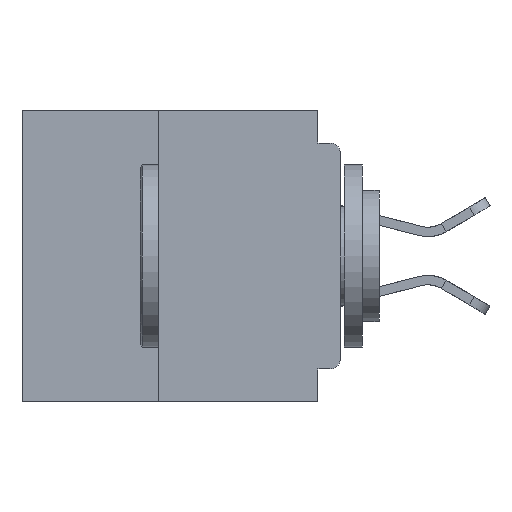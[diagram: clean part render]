
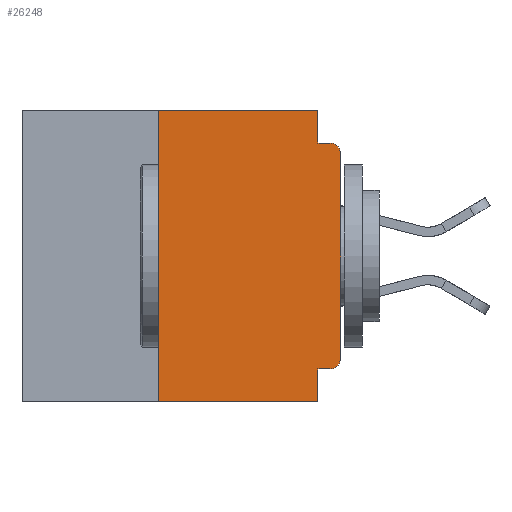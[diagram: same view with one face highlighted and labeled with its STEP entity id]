
A CAD part, left-side view. The second image highlights one B-rep face of the part: STEP entity #26248.
In plain terms, the highlighted planar face has unit normal (-1, 0, 0).
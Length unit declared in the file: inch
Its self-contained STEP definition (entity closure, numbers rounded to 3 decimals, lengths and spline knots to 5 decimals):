
#194 = CARTESIAN_POINT ( 'NONE',  ( 0., 0.031, 0. ) ) ;
#1100 = EDGE_CURVE ( 'NONE', #18490, #32679, #35840, .T. ) ;
#1184 = CARTESIAN_POINT ( 'NONE',  ( 0., 0.031, -0.355 ) ) ;
#1563 = LINE ( 'NONE', #12552, #19149 ) ;
#1639 = EDGE_CURVE ( 'NONE', #33108, #32679, #39386, .T. ) ;
#1641 = DIRECTION ( 'NONE',  ( 0., 0., 1. ) ) ;
#1700 = CIRCLE ( 'NONE', #5880, 0.015 ) ;
#2283 = AXIS2_PLACEMENT_3D ( 'NONE', #19718, #26554, #42294 ) ;
#2343 = EDGE_LOOP ( 'NONE', ( #5915, #18341, #32738, #18912, #7862, #12499, #14066, #38312, #11732, #7358 ) ) ;
#3654 = CARTESIAN_POINT ( 'NONE',  ( 0., 0., -0.06 ) ) ;
#3846 = EDGE_CURVE ( 'NONE', #9332, #11466, #1563, .T. ) ;
#4292 = LINE ( 'NONE', #27196, #38359 ) ;
#5550 = LINE ( 'NONE', #24777, #30886 ) ;
#5880 = AXIS2_PLACEMENT_3D ( 'NONE', #35797, #16117, #39102 ) ;
#5915 = ORIENTED_EDGE ( 'NONE', *, *, #14780, .T. ) ;
#7035 = LINE ( 'NONE', #39237, #15912 ) ;
#7358 = ORIENTED_EDGE ( 'NONE', *, *, #35491, .T. ) ;
#7862 = ORIENTED_EDGE ( 'NONE', *, *, #12087, .F. ) ;
#8947 = VECTOR ( 'NONE', #26849, 39.37008 ) ;
#9332 = VERTEX_POINT ( 'NONE', #1184 ) ;
#9458 = DIRECTION ( 'NONE',  ( 0., 0., 1. ) ) ;
#10410 = PLANE ( 'NONE',  #27218 ) ;
#10957 = CARTESIAN_POINT ( 'NONE',  ( 0., 0.031, -0.4 ) ) ;
#11466 = VERTEX_POINT ( 'NONE', #10957 ) ;
#11732 = ORIENTED_EDGE ( 'NONE', *, *, #21743, .F. ) ;
#12087 = EDGE_CURVE ( 'NONE', #29320, #14224, #4292, .T. ) ;
#12499 = ORIENTED_EDGE ( 'NONE', *, *, #17638, .F. ) ;
#12512 = DIRECTION ( 'NONE',  ( 0., 0., -1. ) ) ;
#12552 = CARTESIAN_POINT ( 'NONE',  ( 0., 0.031, -0.4 ) ) ;
#13156 = VERTEX_POINT ( 'NONE', #13711 ) ;
#13530 = CARTESIAN_POINT ( 'NONE',  ( 0., 0.015, -0.355 ) ) ;
#13711 = CARTESIAN_POINT ( 'NONE',  ( 0., 0.25, -0.4 ) ) ;
#14066 = ORIENTED_EDGE ( 'NONE', *, *, #33616, .T. ) ;
#14224 = VERTEX_POINT ( 'NONE', #194 ) ;
#14371 = CARTESIAN_POINT ( 'NONE',  ( 0., 0., -0.045 ) ) ;
#14440 = CARTESIAN_POINT ( 'NONE',  ( 0., 0.015, -0.045 ) ) ;
#14780 = EDGE_CURVE ( 'NONE', #29279, #33108, #21918, .T. ) ;
#15247 = DIRECTION ( 'NONE',  ( 0., -1., 0. ) ) ;
#15912 = VECTOR ( 'NONE', #32610, 39.37008 ) ;
#16117 = DIRECTION ( 'NONE',  ( -1., 0., 0. ) ) ;
#17638 = EDGE_CURVE ( 'NONE', #13156, #29320, #5550, .T. ) ;
#18341 = ORIENTED_EDGE ( 'NONE', *, *, #1639, .T. ) ;
#18490 = VERTEX_POINT ( 'NONE', #29589 ) ;
#18912 = ORIENTED_EDGE ( 'NONE', *, *, #32392, .F. ) ;
#19149 = VECTOR ( 'NONE', #12512, 39.37008 ) ;
#19339 = CARTESIAN_POINT ( 'NONE',  ( 0., 0., 0. ) ) ;
#19470 = CARTESIAN_POINT ( 'NONE',  ( 0., 0.031, 0. ) ) ;
#19718 = CARTESIAN_POINT ( 'NONE',  ( 0., 0.015, -0.06 ) ) ;
#20393 = DIRECTION ( 'NONE',  ( 0., 0., -1. ) ) ;
#20859 = VECTOR ( 'NONE', #9458, 39.37008 ) ;
#21743 = EDGE_CURVE ( 'NONE', #27913, #9332, #35292, .T. ) ;
#21918 = LINE ( 'NONE', #19339, #20859 ) ;
#22823 = DIRECTION ( 'NONE',  ( 0., 0., -1. ) ) ;
#23584 = CARTESIAN_POINT ( 'NONE',  ( 0., 0., -0.355 ) ) ;
#24416 = CARTESIAN_POINT ( 'NONE',  ( 0., 0., -0.34 ) ) ;
#24777 = CARTESIAN_POINT ( 'NONE',  ( 0., 0.25, -0.4 ) ) ;
#26079 = VECTOR ( 'NONE', #15247, 39.37008 ) ;
#26248 = ADVANCED_FACE ( 'NONE', ( #42129 ), #10410, .F. ) ;
#26554 = DIRECTION ( 'NONE',  ( -1., 0., 0. ) ) ;
#26849 = DIRECTION ( 'NONE',  ( 0., 1., 0. ) ) ;
#27196 = CARTESIAN_POINT ( 'NONE',  ( 0., 0.437, 0. ) ) ;
#27218 = AXIS2_PLACEMENT_3D ( 'NONE', #36809, #40098, #20393 ) ;
#27913 = VERTEX_POINT ( 'NONE', #13530 ) ;
#29279 = VERTEX_POINT ( 'NONE', #24416 ) ;
#29320 = VERTEX_POINT ( 'NONE', #37760 ) ;
#29589 = CARTESIAN_POINT ( 'NONE',  ( 0., 0.031, -0.045 ) ) ;
#30511 = DIRECTION ( 'NONE',  ( 0., -1., 0. ) ) ;
#30886 = VECTOR ( 'NONE', #1641, 39.37008 ) ;
#32392 = EDGE_CURVE ( 'NONE', #14224, #18490, #36371, .T. ) ;
#32610 = DIRECTION ( 'NONE',  ( 0., -1., 0. ) ) ;
#32679 = VERTEX_POINT ( 'NONE', #14440 ) ;
#32738 = ORIENTED_EDGE ( 'NONE', *, *, #1100, .F. ) ;
#33108 = VERTEX_POINT ( 'NONE', #3654 ) ;
#33616 = EDGE_CURVE ( 'NONE', #13156, #11466, #7035, .T. ) ;
#34319 = VECTOR ( 'NONE', #22823, 39.37008 ) ;
#35292 = LINE ( 'NONE', #23584, #8947 ) ;
#35491 = EDGE_CURVE ( 'NONE', #27913, #29279, #1700, .T. ) ;
#35797 = CARTESIAN_POINT ( 'NONE',  ( 0., 0.015, -0.34 ) ) ;
#35840 = LINE ( 'NONE', #14371, #26079 ) ;
#36371 = LINE ( 'NONE', #19470, #34319 ) ;
#36809 = CARTESIAN_POINT ( 'NONE',  ( 0., 0.437, 0. ) ) ;
#37760 = CARTESIAN_POINT ( 'NONE',  ( 0., 0.25, 0. ) ) ;
#38312 = ORIENTED_EDGE ( 'NONE', *, *, #3846, .F. ) ;
#38359 = VECTOR ( 'NONE', #30511, 39.37008 ) ;
#39102 = DIRECTION ( 'NONE',  ( 0., 0., -1. ) ) ;
#39237 = CARTESIAN_POINT ( 'NONE',  ( 0., 0.437, -0.4 ) ) ;
#39386 = CIRCLE ( 'NONE', #2283, 0.015 ) ;
#40098 = DIRECTION ( 'NONE',  ( 1., 0., 0. ) ) ;
#42129 = FACE_OUTER_BOUND ( 'NONE', #2343, .T. ) ;
#42294 = DIRECTION ( 'NONE',  ( 0., 0., -1. ) ) ;
